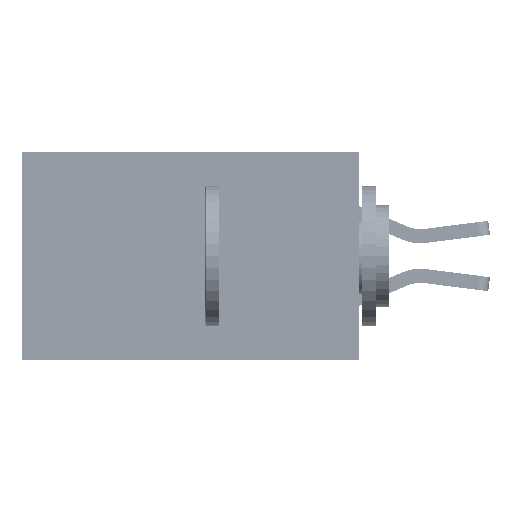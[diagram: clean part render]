
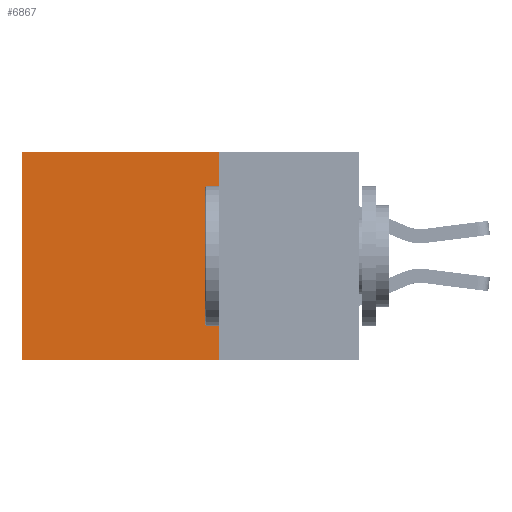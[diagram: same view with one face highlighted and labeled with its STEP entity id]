
A CAD part, left-side view. The second image highlights one B-rep face of the part: STEP entity #6867.
In plain terms, the highlighted planar face has unit normal (-1, 0, 0).
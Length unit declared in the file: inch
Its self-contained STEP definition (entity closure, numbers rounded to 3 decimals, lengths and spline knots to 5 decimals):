
#156 = PLANE ( 'NONE',  #51419 ) ;
#2690 = DIRECTION ( 'NONE',  ( 0., 1., 0. ) ) ;
#3588 = CARTESIAN_POINT ( 'NONE',  ( 0.2875, 0.25, 0. ) ) ;
#4569 = CARTESIAN_POINT ( 'NONE',  ( 0.2875, 0.25, 0. ) ) ;
#5277 = CARTESIAN_POINT ( 'NONE',  ( 0.2875, 0.25, -0.37 ) ) ;
#6867 = ADVANCED_FACE ( 'NONE', ( #16108 ), #156, .F. ) ;
#7818 = VECTOR ( 'NONE', #40589, 39.37008 ) ;
#8083 = CARTESIAN_POINT ( 'NONE',  ( 0.2875, 0.6, 0. ) ) ;
#9009 = DIRECTION ( 'NONE',  ( 0., 0., -1. ) ) ;
#9024 = ORIENTED_EDGE ( 'NONE', *, *, #13392, .T. ) ;
#13116 = VECTOR ( 'NONE', #2690, 39.37008 ) ;
#13205 = CARTESIAN_POINT ( 'NONE',  ( 0.2875, 0.25, 0. ) ) ;
#13246 = ORIENTED_EDGE ( 'NONE', *, *, #22362, .F. ) ;
#13392 = EDGE_CURVE ( 'NONE', #36943, #41680, #50039, .T. ) ;
#15560 = CARTESIAN_POINT ( 'NONE',  ( 0.2875, 0.6, 0. ) ) ;
#16108 = FACE_OUTER_BOUND ( 'NONE', #44573, .T. ) ;
#18722 = LINE ( 'NONE', #3588, #13116 ) ;
#22362 = EDGE_CURVE ( 'NONE', #33743, #41680, #22662, .T. ) ;
#22662 = LINE ( 'NONE', #5277, #46880 ) ;
#23993 = EDGE_CURVE ( 'NONE', #33077, #36943, #18722, .T. ) ;
#24927 = DIRECTION ( 'NONE',  ( 1., 0., 0. ) ) ;
#27877 = CARTESIAN_POINT ( 'NONE',  ( 0.2875, 0.6, -0.37 ) ) ;
#31417 = CARTESIAN_POINT ( 'NONE',  ( 0.2875, 0.25, -0.37 ) ) ;
#33077 = VERTEX_POINT ( 'NONE', #46292 ) ;
#33743 = VERTEX_POINT ( 'NONE', #31417 ) ;
#36943 = VERTEX_POINT ( 'NONE', #15560 ) ;
#37328 = ORIENTED_EDGE ( 'NONE', *, *, #23993, .T. ) ;
#37713 = LINE ( 'NONE', #4569, #7818 ) ;
#39998 = EDGE_CURVE ( 'NONE', #33077, #33743, #37713, .T. ) ;
#40589 = DIRECTION ( 'NONE',  ( 0., 0., -1. ) ) ;
#40996 = ORIENTED_EDGE ( 'NONE', *, *, #39998, .F. ) ;
#41680 = VERTEX_POINT ( 'NONE', #27877 ) ;
#44573 = EDGE_LOOP ( 'NONE', ( #9024, #13246, #40996, #37328 ) ) ;
#46292 = CARTESIAN_POINT ( 'NONE',  ( 0.2875, 0.25, 0. ) ) ;
#46880 = VECTOR ( 'NONE', #48919, 39.37008 ) ;
#47765 = DIRECTION ( 'NONE',  ( 0., 0., -1. ) ) ;
#48919 = DIRECTION ( 'NONE',  ( 0., 1., 0. ) ) ;
#49423 = VECTOR ( 'NONE', #47765, 39.37008 ) ;
#50039 = LINE ( 'NONE', #8083, #49423 ) ;
#51419 = AXIS2_PLACEMENT_3D ( 'NONE', #13205, #24927, #9009 ) ;
